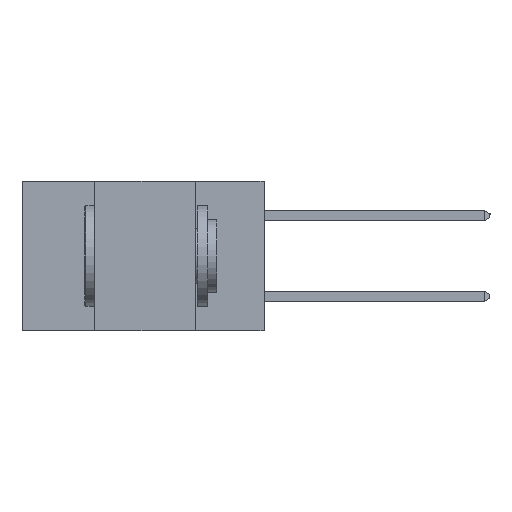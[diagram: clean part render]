
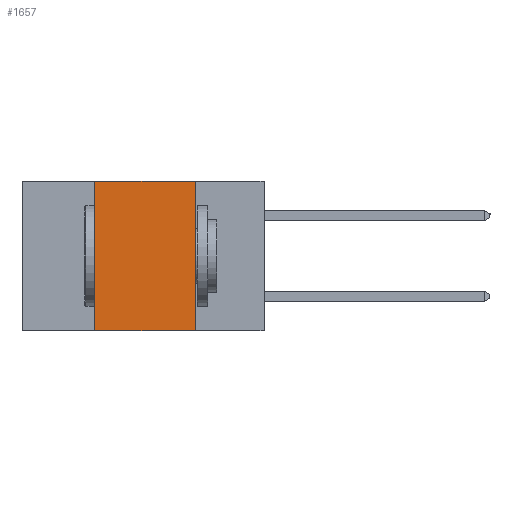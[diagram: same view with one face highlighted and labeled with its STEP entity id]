
A CAD part, left-side view. The second image highlights one B-rep face of the part: STEP entity #1657.
In plain terms, the highlighted planar face has unit normal (-1, 0, 0).
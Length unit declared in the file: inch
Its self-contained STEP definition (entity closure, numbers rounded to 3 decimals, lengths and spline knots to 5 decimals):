
#98 = EDGE_CURVE ( 'NONE', #4772, #2478, #8368, .T. ) ;
#986 = DIRECTION ( 'NONE',  ( 0., 0., -1. ) ) ;
#1080 = CARTESIAN_POINT ( 'NONE',  ( 0., 0.42, -0.37 ) ) ;
#1108 = EDGE_CURVE ( 'NONE', #4772, #12353, #12487, .T. ) ;
#1657 = ADVANCED_FACE ( 'NONE', ( #11329 ), #5877, .F. ) ;
#2294 = CARTESIAN_POINT ( 'NONE',  ( 0., 0.6, 0. ) ) ;
#2319 = VECTOR ( 'NONE', #12862, 39.37008 ) ;
#2478 = VERTEX_POINT ( 'NONE', #5303 ) ;
#2532 = CARTESIAN_POINT ( 'NONE',  ( 0., 0.42, -0.37 ) ) ;
#3312 = VECTOR ( 'NONE', #6714, 39.37008 ) ;
#3477 = VECTOR ( 'NONE', #13023, 39.37008 ) ;
#3479 = VERTEX_POINT ( 'NONE', #12087 ) ;
#4373 = ORIENTED_EDGE ( 'NONE', *, *, #98, .F. ) ;
#4772 = VERTEX_POINT ( 'NONE', #1080 ) ;
#5115 = ORIENTED_EDGE ( 'NONE', *, *, #1108, .T. ) ;
#5303 = CARTESIAN_POINT ( 'NONE',  ( 0., 0.42, 0. ) ) ;
#5306 = AXIS2_PLACEMENT_3D ( 'NONE', #2294, #10485, #986 ) ;
#5877 = PLANE ( 'NONE',  #5306 ) ;
#6626 = EDGE_CURVE ( 'NONE', #2478, #3479, #7310, .T. ) ;
#6681 = CARTESIAN_POINT ( 'NONE',  ( 0., 0.17, -0.37 ) ) ;
#6714 = DIRECTION ( 'NONE',  ( 0., 0., -1. ) ) ;
#7310 = LINE ( 'NONE', #8292, #2319 ) ;
#7398 = EDGE_CURVE ( 'NONE', #3479, #12353, #14588, .T. ) ;
#7993 = CARTESIAN_POINT ( 'NONE',  ( 0., 0.17, -0.37 ) ) ;
#8292 = CARTESIAN_POINT ( 'NONE',  ( 0., 0.6, 0. ) ) ;
#8368 = LINE ( 'NONE', #2532, #3477 ) ;
#8747 = DIRECTION ( 'NONE',  ( 0., -1., 0. ) ) ;
#8985 = VECTOR ( 'NONE', #8747, 39.37008 ) ;
#9756 = ORIENTED_EDGE ( 'NONE', *, *, #6626, .F. ) ;
#10485 = DIRECTION ( 'NONE',  ( 1., 0., 0. ) ) ;
#11329 = FACE_OUTER_BOUND ( 'NONE', #12077, .T. ) ;
#12077 = EDGE_LOOP ( 'NONE', ( #13379, #9756, #4373, #5115 ) ) ;
#12087 = CARTESIAN_POINT ( 'NONE',  ( 0., 0.17, 0. ) ) ;
#12353 = VERTEX_POINT ( 'NONE', #6681 ) ;
#12487 = LINE ( 'NONE', #13480, #8985 ) ;
#12862 = DIRECTION ( 'NONE',  ( 0., -1., 0. ) ) ;
#13023 = DIRECTION ( 'NONE',  ( 0., 0., 1. ) ) ;
#13379 = ORIENTED_EDGE ( 'NONE', *, *, #7398, .F. ) ;
#13480 = CARTESIAN_POINT ( 'NONE',  ( 0., 0.6, -0.37 ) ) ;
#14588 = LINE ( 'NONE', #7993, #3312 ) ;
